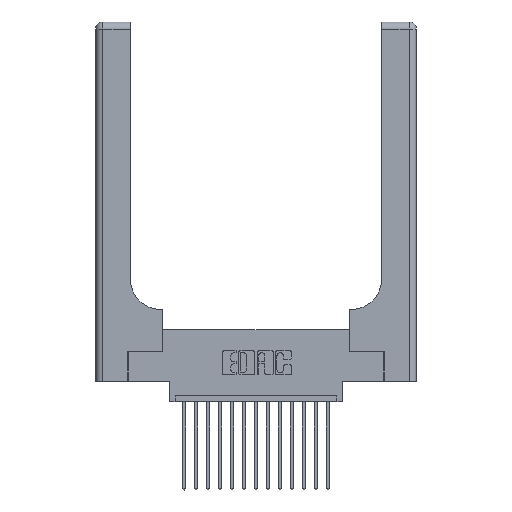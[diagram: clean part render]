
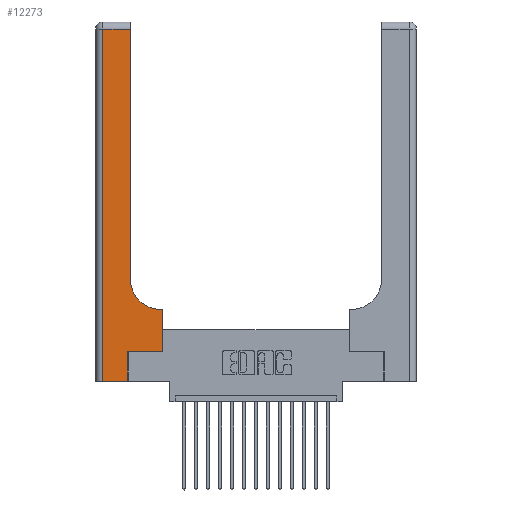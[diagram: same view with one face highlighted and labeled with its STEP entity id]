
A CAD part, top view. The second image highlights one B-rep face of the part: STEP entity #12273.
In plain terms, the highlighted planar face has unit normal (0, 0, 1).
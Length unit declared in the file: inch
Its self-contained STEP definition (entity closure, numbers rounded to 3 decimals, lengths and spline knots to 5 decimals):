
#214 = VERTEX_POINT ( 'NONE', #15998 ) ;
#366 = LINE ( 'NONE', #3911, #12787 ) ;
#387 = CARTESIAN_POINT ( 'NONE',  ( 0.2915, 0.6, 0.37 ) ) ;
#533 = ORIENTED_EDGE ( 'NONE', *, *, #2796, .T. ) ;
#672 = EDGE_CURVE ( 'NONE', #214, #18192, #6552, .T. ) ;
#924 = EDGE_CURVE ( 'NONE', #12460, #2716, #13430, .T. ) ;
#1006 = DIRECTION ( 'NONE',  ( -1., 0., 0. ) ) ;
#1118 = CARTESIAN_POINT ( 'NONE',  ( 0.5585, 0.6, 0.37 ) ) ;
#1171 = DIRECTION ( 'NONE',  ( 0., 1., 0. ) ) ;
#2162 = LINE ( 'NONE', #5536, #13408 ) ;
#2577 = VECTOR ( 'NONE', #11630, 39.37008 ) ;
#2716 = VERTEX_POINT ( 'NONE', #14516 ) ;
#2796 = EDGE_CURVE ( 'NONE', #8979, #214, #11964, .T. ) ;
#2833 = EDGE_CURVE ( 'NONE', #2716, #3581, #9465, .T. ) ;
#2904 = CARTESIAN_POINT ( 'NONE',  ( 0.06, 3., 0.37 ) ) ;
#3334 = CARTESIAN_POINT ( 'NONE',  ( 0.2915, 2.94, 0.37 ) ) ;
#3581 = VERTEX_POINT ( 'NONE', #12678 ) ;
#3648 = ORIENTED_EDGE ( 'NONE', *, *, #8967, .T. ) ;
#3895 = VERTEX_POINT ( 'NONE', #12471 ) ;
#3911 = CARTESIAN_POINT ( 'NONE',  ( 0.5585, 0.25, 0.37 ) ) ;
#4358 = DIRECTION ( 'NONE',  ( 0., 1., 0. ) ) ;
#4546 = LINE ( 'NONE', #18771, #4992 ) ;
#4992 = VECTOR ( 'NONE', #1171, 39.37008 ) ;
#5340 = ORIENTED_EDGE ( 'NONE', *, *, #15951, .T. ) ;
#5536 = CARTESIAN_POINT ( 'NONE',  ( 0., 2.94, 0.37 ) ) ;
#5676 = DIRECTION ( 'NONE',  ( -1., 0., 0. ) ) ;
#5762 = EDGE_LOOP ( 'NONE', ( #6525, #5340, #533, #7685, #3648, #9040, #12585, #13768, #12536 ) ) ;
#6061 = DIRECTION ( 'NONE',  ( 1., 0., 0. ) ) ;
#6127 = DIRECTION ( 'NONE',  ( 1., 0., 0. ) ) ;
#6129 = DIRECTION ( 'NONE',  ( 1., 0., 0. ) ) ;
#6525 = ORIENTED_EDGE ( 'NONE', *, *, #12714, .T. ) ;
#6552 = LINE ( 'NONE', #7149, #14125 ) ;
#6742 = DIRECTION ( 'NONE',  ( 0., 0., -1. ) ) ;
#6801 = CARTESIAN_POINT ( 'NONE',  ( 0., 3., 0.37 ) ) ;
#6930 = DIRECTION ( 'NONE',  ( 0., 1., 0. ) ) ;
#7149 = CARTESIAN_POINT ( 'NONE',  ( 0., 0., 0.37 ) ) ;
#7685 = ORIENTED_EDGE ( 'NONE', *, *, #672, .T. ) ;
#7712 = DIRECTION ( 'NONE',  ( 0., 0., -1. ) ) ;
#8010 = EDGE_CURVE ( 'NONE', #3895, #12460, #366, .T. ) ;
#8771 = CARTESIAN_POINT ( 'NONE',  ( 0.5415, 0.85, 0.37 ) ) ;
#8967 = EDGE_CURVE ( 'NONE', #18192, #17855, #16415, .T. ) ;
#8979 = VERTEX_POINT ( 'NONE', #11601 ) ;
#9040 = ORIENTED_EDGE ( 'NONE', *, *, #10767, .T. ) ;
#9131 = CARTESIAN_POINT ( 'NONE',  ( 0.269, 0.25, 0.37 ) ) ;
#9465 = CIRCLE ( 'NONE', #10963, 0.25 ) ;
#9539 = VECTOR ( 'NONE', #18045, 39.37008 ) ;
#9830 = PLANE ( 'NONE',  #12092 ) ;
#10767 = EDGE_CURVE ( 'NONE', #17855, #3895, #14259, .T. ) ;
#10963 = AXIS2_PLACEMENT_3D ( 'NONE', #8771, #7712, #6127 ) ;
#11328 = CARTESIAN_POINT ( 'NONE',  ( 0.269, 0., 0.37 ) ) ;
#11601 = CARTESIAN_POINT ( 'NONE',  ( 0.06, 2.94, 0.37 ) ) ;
#11630 = DIRECTION ( 'NONE',  ( 0., -1., 0. ) ) ;
#11683 = FACE_OUTER_BOUND ( 'NONE', #5762, .T. ) ;
#11718 = CARTESIAN_POINT ( 'NONE',  ( 0.269, 0., 0.37 ) ) ;
#11964 = LINE ( 'NONE', #2904, #2577 ) ;
#12033 = VERTEX_POINT ( 'NONE', #3334 ) ;
#12092 = AXIS2_PLACEMENT_3D ( 'NONE', #6801, #6742, #1006 ) ;
#12273 = ADVANCED_FACE ( 'NONE', ( #11683 ), #9830, .F. ) ;
#12460 = VERTEX_POINT ( 'NONE', #1118 ) ;
#12471 = CARTESIAN_POINT ( 'NONE',  ( 0.5585, 0.25, 0.37 ) ) ;
#12536 = ORIENTED_EDGE ( 'NONE', *, *, #2833, .T. ) ;
#12585 = ORIENTED_EDGE ( 'NONE', *, *, #8010, .T. ) ;
#12678 = CARTESIAN_POINT ( 'NONE',  ( 0.2915, 0.85, 0.37 ) ) ;
#12714 = EDGE_CURVE ( 'NONE', #3581, #12033, #4546, .T. ) ;
#12787 = VECTOR ( 'NONE', #6930, 39.37008 ) ;
#13408 = VECTOR ( 'NONE', #5676, 39.37008 ) ;
#13430 = LINE ( 'NONE', #387, #9539 ) ;
#13768 = ORIENTED_EDGE ( 'NONE', *, *, #924, .T. ) ;
#14104 = VECTOR ( 'NONE', #4358, 39.37008 ) ;
#14125 = VECTOR ( 'NONE', #6061, 39.37008 ) ;
#14259 = LINE ( 'NONE', #9131, #16131 ) ;
#14516 = CARTESIAN_POINT ( 'NONE',  ( 0.5415, 0.6, 0.37 ) ) ;
#15852 = CARTESIAN_POINT ( 'NONE',  ( 0.269, 0.25, 0.37 ) ) ;
#15951 = EDGE_CURVE ( 'NONE', #12033, #8979, #2162, .T. ) ;
#15998 = CARTESIAN_POINT ( 'NONE',  ( 0.06, 0., 0.37 ) ) ;
#16131 = VECTOR ( 'NONE', #6129, 39.37008 ) ;
#16415 = LINE ( 'NONE', #11718, #14104 ) ;
#17855 = VERTEX_POINT ( 'NONE', #15852 ) ;
#18045 = DIRECTION ( 'NONE',  ( -1., 0., 0. ) ) ;
#18192 = VERTEX_POINT ( 'NONE', #11328 ) ;
#18771 = CARTESIAN_POINT ( 'NONE',  ( 0.2915, 3., 0.37 ) ) ;
